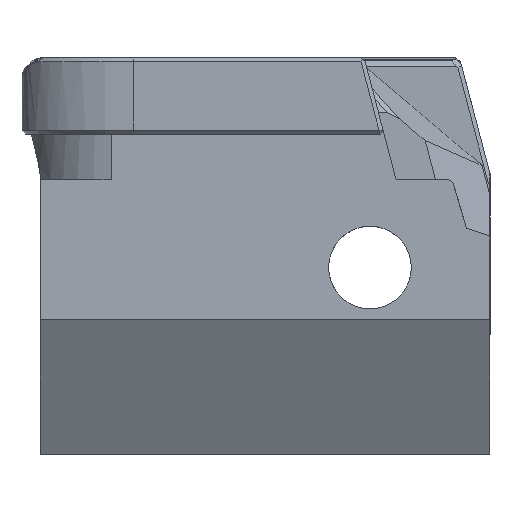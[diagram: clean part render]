
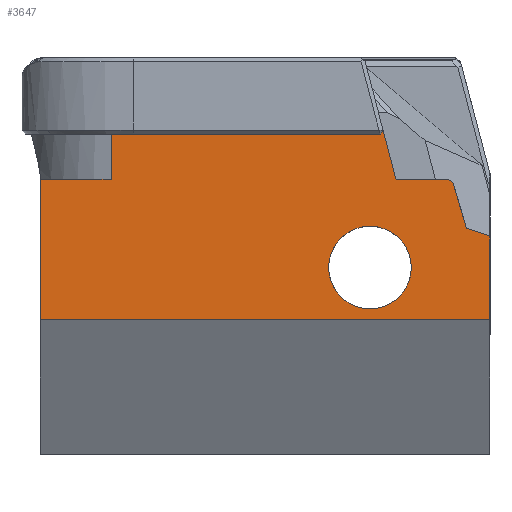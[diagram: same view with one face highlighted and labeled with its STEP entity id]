
A CAD part, front view. The second image highlights one B-rep face of the part: STEP entity #3647.
In plain terms, the highlighted planar face has unit normal (0, -1, 0).
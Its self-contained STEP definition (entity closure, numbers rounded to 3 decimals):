
#15 = CARTESIAN_POINT ( 'NONE',  ( -71.374, 60.85, -0.1 ) ) ;
#27 = DIRECTION ( 'NONE',  ( 0., 0., 1. ) ) ;
#31 = CARTESIAN_POINT ( 'NONE',  ( -93.746, 60.85, 2.75 ) ) ;
#128 = EDGE_LOOP ( 'NONE', ( #2581, #1050 ) ) ;
#172 = CARTESIAN_POINT ( 'NONE',  ( -68.101, 60.85, -0.1 ) ) ;
#184 = EDGE_CURVE ( 'NONE', #4258, #728, #3385, .T. ) ;
#199 = CARTESIAN_POINT ( 'NONE',  ( -67.78, 60.85, -0.34 ) ) ;
#268 = CARTESIAN_POINT ( 'NONE',  ( -70.172, 60.85, -0.1 ) ) ;
#309 = EDGE_CURVE ( 'NONE', #2322, #4125, #2274, .T. ) ;
#372 = CARTESIAN_POINT ( 'NONE',  ( -70.413, 60.85, -5.65 ) ) ;
#563 = VECTOR ( 'NONE', #5201, 1000. ) ;
#584 = DIRECTION ( 'NONE',  ( -1., 0., 0. ) ) ;
#610 = CARTESIAN_POINT ( 'NONE',  ( 104.021, 60.85, 2.75 ) ) ;
#701 = ORIENTED_EDGE ( 'NONE', *, *, #4624, .T. ) ;
#711 = CIRCLE ( 'NONE', #1645, 2.6 ) ;
#728 = VERTEX_POINT ( 'NONE', #2083 ) ;
#743 = VERTEX_POINT ( 'NONE', #199 ) ;
#850 = VERTEX_POINT ( 'NONE', #1106 ) ;
#1050 = ORIENTED_EDGE ( 'NONE', *, *, #3028, .F. ) ;
#1106 = CARTESIAN_POINT ( 'NONE',  ( -65.464, 60.85, -3.663 ) ) ;
#1311 = VERTEX_POINT ( 'NONE', #1652 ) ;
#1368 = EDGE_LOOP ( 'NONE', ( #1471, #5082, #2361, #3247, #4492, #701, #4628, #3843, #2502, #3572, #4635, #4616 ) ) ;
#1402 = DIRECTION ( 'NONE',  ( 0.254, 0., -0.967 ) ) ;
#1471 = ORIENTED_EDGE ( 'NONE', *, *, #184, .T. ) ;
#1500 = LINE ( 'NONE', #2629, #3692 ) ;
#1510 = EDGE_CURVE ( 'NONE', #4832, #1838, #2243, .T. ) ;
#1591 = CARTESIAN_POINT ( 'NONE',  ( -89.297, 60.85, -0.1 ) ) ;
#1645 = AXIS2_PLACEMENT_3D ( 'NONE', #3336, #2250, #2542 ) ;
#1652 = CARTESIAN_POINT ( 'NONE',  ( -75.613, 60.85, -5.65 ) ) ;
#1710 = EDGE_CURVE ( 'NONE', #2851, #850, #5092, .T. ) ;
#1717 = CARTESIAN_POINT ( 'NONE',  ( -93.746, 60.85, -8.934 ) ) ;
#1736 = DIRECTION ( 'NONE',  ( -1., 0., 0. ) ) ;
#1750 = DIRECTION ( 'NONE',  ( 1., 0., 0. ) ) ;
#1838 = VERTEX_POINT ( 'NONE', #15 ) ;
#1924 = CIRCLE ( 'NONE', #2013, 2.6 ) ;
#2013 = AXIS2_PLACEMENT_3D ( 'NONE', #2041, #4080, #27 ) ;
#2037 = LINE ( 'NONE', #2458, #3273 ) ;
#2041 = CARTESIAN_POINT ( 'NONE',  ( -73.013, 60.85, -5.65 ) ) ;
#2083 = CARTESIAN_POINT ( 'NONE',  ( -65.464, 60.85, -8.934 ) ) ;
#2085 = LINE ( 'NONE', #2527, #3184 ) ;
#2134 = CARTESIAN_POINT ( 'NONE',  ( -66.989, 60.85, -3.017 ) ) ;
#2243 = LINE ( 'NONE', #3071, #2817 ) ;
#2250 = DIRECTION ( 'NONE',  ( 0., -1., 0. ) ) ;
#2274 = LINE ( 'NONE', #268, #4081 ) ;
#2276 = EDGE_CURVE ( 'NONE', #2322, #3914, #2037, .T. ) ;
#2306 = AXIS2_PLACEMENT_3D ( 'NONE', #4324, #5161, #2681 ) ;
#2322 = VERTEX_POINT ( 'NONE', #1591 ) ;
#2338 = VECTOR ( 'NONE', #4746, 1000. ) ;
#2348 = EDGE_CURVE ( 'NONE', #743, #2851, #2980, .T. ) ;
#2361 = ORIENTED_EDGE ( 'NONE', *, *, #1710, .F. ) ;
#2458 = CARTESIAN_POINT ( 'NONE',  ( -89.297, 60.85, -0.1 ) ) ;
#2467 = LINE ( 'NONE', #610, #2478 ) ;
#2478 = VECTOR ( 'NONE', #584, 1000. ) ;
#2502 = ORIENTED_EDGE ( 'NONE', *, *, #3808, .T. ) ;
#2515 = EDGE_CURVE ( 'NONE', #743, #4607, #2854, .T. ) ;
#2527 = CARTESIAN_POINT ( 'NONE',  ( -70.172, 60.85, -0.1 ) ) ;
#2542 = DIRECTION ( 'NONE',  ( 0., 0., 1. ) ) ;
#2581 = ORIENTED_EDGE ( 'NONE', *, *, #3450, .F. ) ;
#2584 = VECTOR ( 'NONE', #4923, 1000. ) ;
#2629 = CARTESIAN_POINT ( 'NONE',  ( -6.622, 60.85, 88.043 ) ) ;
#2637 = EDGE_CURVE ( 'NONE', #728, #850, #3696, .T. ) ;
#2681 = DIRECTION ( 'NONE',  ( 0., 0., -1. ) ) ;
#2788 = FACE_OUTER_BOUND ( 'NONE', #1368, .T. ) ;
#2817 = VECTOR ( 'NONE', #1402, 1000. ) ;
#2851 = VERTEX_POINT ( 'NONE', #5221 ) ;
#2854 = LINE ( 'NONE', #3646, #563 ) ;
#2980 = LINE ( 'NONE', #2134, #4882 ) ;
#3028 = EDGE_CURVE ( 'NONE', #1311, #5123, #1924, .T. ) ;
#3071 = CARTESIAN_POINT ( 'NONE',  ( -60.715, 60.85, -40.602 ) ) ;
#3143 = CARTESIAN_POINT ( 'NONE',  ( -72.374, 60.85, 2.75 ) ) ;
#3184 = VECTOR ( 'NONE', #1736, 1000. ) ;
#3247 = ORIENTED_EDGE ( 'NONE', *, *, #2348, .F. ) ;
#3273 = VECTOR ( 'NONE', #4448, 1000. ) ;
#3336 = CARTESIAN_POINT ( 'NONE',  ( -73.013, 60.85, -5.65 ) ) ;
#3384 = CARTESIAN_POINT ( 'NONE',  ( -89.297, 60.85, 2.75 ) ) ;
#3385 = LINE ( 'NONE', #4928, #4162 ) ;
#3422 = CARTESIAN_POINT ( 'NONE',  ( -72.187, 60.85, 2.992 ) ) ;
#3423 = CARTESIAN_POINT ( 'NONE',  ( -56.462, 60.85, -6.597 ) ) ;
#3450 = EDGE_CURVE ( 'NONE', #5123, #1311, #711, .T. ) ;
#3475 = CARTESIAN_POINT ( 'NONE',  ( -65.464, 60.85, 2.75 ) ) ;
#3572 = ORIENTED_EDGE ( 'NONE', *, *, #2276, .F. ) ;
#3634 = CARTESIAN_POINT ( 'NONE',  ( -93.746, 60.85, -0.1 ) ) ;
#3646 = CARTESIAN_POINT ( 'NONE',  ( -68.101, 60.85, -0.1 ) ) ;
#3647 = ADVANCED_FACE ( 'NONE', ( #2788, #4349 ), #3893, .T. ) ;
#3657 = LINE ( 'NONE', #31, #2584 ) ;
#3692 = VECTOR ( 'NONE', #4225, 1000. ) ;
#3696 = LINE ( 'NONE', #3475, #2338 ) ;
#3808 = EDGE_CURVE ( 'NONE', #4317, #3914, #2467, .T. ) ;
#3810 = DIRECTION ( 'NONE',  ( -1., 0., 0. ) ) ;
#3843 = ORIENTED_EDGE ( 'NONE', *, *, #4744, .F. ) ;
#3893 = PLANE ( 'NONE',  #2306 ) ;
#3914 = VERTEX_POINT ( 'NONE', #3384 ) ;
#4080 = DIRECTION ( 'NONE',  ( 0., -1., 0. ) ) ;
#4081 = VECTOR ( 'NONE', #3810, 1000. ) ;
#4125 = VERTEX_POINT ( 'NONE', #3634 ) ;
#4162 = VECTOR ( 'NONE', #1750, 1000. ) ;
#4225 = DIRECTION ( 'NONE',  ( 0.611, 0., 0.792 ) ) ;
#4258 = VERTEX_POINT ( 'NONE', #1717 ) ;
#4317 = VERTEX_POINT ( 'NONE', #3143 ) ;
#4324 = CARTESIAN_POINT ( 'NONE',  ( 104.021, 60.85, 2.75 ) ) ;
#4349 = FACE_BOUND ( 'NONE', #128, .T. ) ;
#4448 = DIRECTION ( 'NONE',  ( 0., 0., 1. ) ) ;
#4492 = ORIENTED_EDGE ( 'NONE', *, *, #2515, .T. ) ;
#4602 = DIRECTION ( 'NONE',  ( 0.283, 0., -0.959 ) ) ;
#4607 = VERTEX_POINT ( 'NONE', #172 ) ;
#4616 = ORIENTED_EDGE ( 'NONE', *, *, #5166, .T. ) ;
#4624 = EDGE_CURVE ( 'NONE', #4607, #1838, #2085, .T. ) ;
#4628 = ORIENTED_EDGE ( 'NONE', *, *, #1510, .F. ) ;
#4635 = ORIENTED_EDGE ( 'NONE', *, *, #309, .T. ) ;
#4728 = DIRECTION ( 'NONE',  ( 0.951, 0., -0.31 ) ) ;
#4744 = EDGE_CURVE ( 'NONE', #4317, #4832, #1500, .T. ) ;
#4746 = DIRECTION ( 'NONE',  ( 0., 0., 1. ) ) ;
#4832 = VERTEX_POINT ( 'NONE', #3422 ) ;
#4882 = VECTOR ( 'NONE', #4602, 1000. ) ;
#4923 = DIRECTION ( 'NONE',  ( 0., 0., -1. ) ) ;
#4928 = CARTESIAN_POINT ( 'NONE',  ( -185.4, 60.85, -8.934 ) ) ;
#4955 = VECTOR ( 'NONE', #4728, 1000. ) ;
#5082 = ORIENTED_EDGE ( 'NONE', *, *, #2637, .T. ) ;
#5092 = LINE ( 'NONE', #3423, #4955 ) ;
#5123 = VERTEX_POINT ( 'NONE', #372 ) ;
#5161 = DIRECTION ( 'NONE',  ( 0., -1., 0. ) ) ;
#5166 = EDGE_CURVE ( 'NONE', #4125, #4258, #3657, .T. ) ;
#5201 = DIRECTION ( 'NONE',  ( -0.801, 0., 0.599 ) ) ;
#5221 = CARTESIAN_POINT ( 'NONE',  ( -66.94, 60.85, -3.182 ) ) ;
